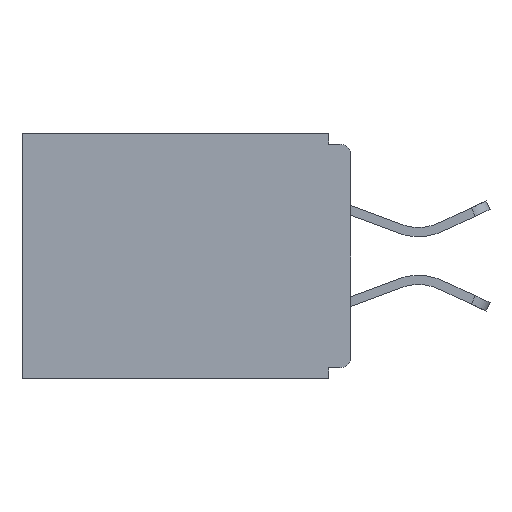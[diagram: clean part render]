
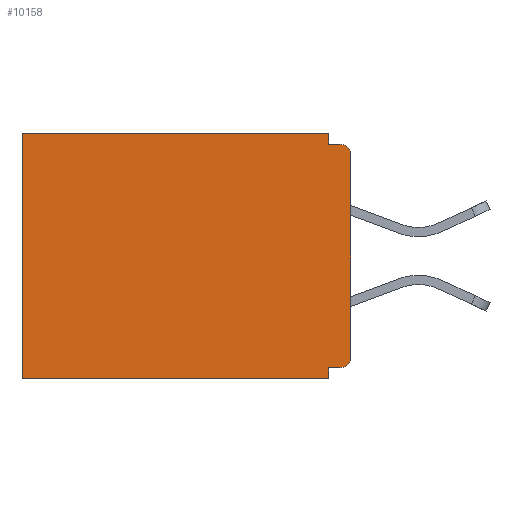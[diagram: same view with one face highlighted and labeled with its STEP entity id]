
A CAD part, left-side view. The second image highlights one B-rep face of the part: STEP entity #10158.
In plain terms, the highlighted planar face has unit normal (-1, 0, 0).
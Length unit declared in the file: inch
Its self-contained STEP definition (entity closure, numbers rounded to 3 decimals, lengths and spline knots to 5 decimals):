
#360 = CARTESIAN_POINT ( 'NONE',  ( 0.298, 0.031, -0.343 ) ) ;
#511 = VERTEX_POINT ( 'NONE', #20464 ) ;
#1311 = CARTESIAN_POINT ( 'NONE',  ( 0.298, 0., -0.328 ) ) ;
#1667 = DIRECTION ( 'NONE',  ( 1., 0., 0. ) ) ;
#1739 = CARTESIAN_POINT ( 'NONE',  ( 0.298, 0., -0.015 ) ) ;
#2010 = LINE ( 'NONE', #12875, #14584 ) ;
#2034 = VECTOR ( 'NONE', #11067, 39.37008 ) ;
#2295 = AXIS2_PLACEMENT_3D ( 'NONE', #22097, #24158, #23992 ) ;
#2498 = CARTESIAN_POINT ( 'NONE',  ( 0.298, 0.46, -0.343 ) ) ;
#2510 = FACE_OUTER_BOUND ( 'NONE', #4652, .T. ) ;
#2624 = CARTESIAN_POINT ( 'NONE',  ( 0.298, 0., -0.03 ) ) ;
#2824 = VERTEX_POINT ( 'NONE', #17046 ) ;
#2877 = LINE ( 'NONE', #1739, #2034 ) ;
#2881 = LINE ( 'NONE', #17395, #10744 ) ;
#2936 = VERTEX_POINT ( 'NONE', #21156 ) ;
#3415 = ORIENTED_EDGE ( 'NONE', *, *, #20116, .F. ) ;
#3960 = CIRCLE ( 'NONE', #19292, 0.015 ) ;
#4278 = EDGE_CURVE ( 'NONE', #511, #17230, #2881, .T. ) ;
#4652 = EDGE_LOOP ( 'NONE', ( #11288, #8865, #23082, #16800, #13172, #14732, #3415, #10312, #14212, #19176 ) ) ;
#4686 = DIRECTION ( 'NONE',  ( 0., 0., -1. ) ) ;
#5114 = VECTOR ( 'NONE', #4686, 39.37008 ) ;
#5478 = CARTESIAN_POINT ( 'NONE',  ( 0.298, 0.46, 0. ) ) ;
#5620 = VERTEX_POINT ( 'NONE', #2498 ) ;
#7881 = DIRECTION ( 'NONE',  ( 0., 0., -1. ) ) ;
#8030 = VERTEX_POINT ( 'NONE', #2624 ) ;
#8452 = CARTESIAN_POINT ( 'NONE',  ( 0.298, 0.031, -0.343 ) ) ;
#8865 = ORIENTED_EDGE ( 'NONE', *, *, #14608, .F. ) ;
#9141 = VECTOR ( 'NONE', #23404, 39.37008 ) ;
#10158 = ADVANCED_FACE ( 'NONE', ( #2510 ), #24097, .F. ) ;
#10312 = ORIENTED_EDGE ( 'NONE', *, *, #14454, .F. ) ;
#10385 = EDGE_CURVE ( 'NONE', #2936, #2824, #15359, .T. ) ;
#10394 = DIRECTION ( 'NONE',  ( 0., 1., 0. ) ) ;
#10738 = EDGE_CURVE ( 'NONE', #17230, #5620, #23297, .T. ) ;
#10744 = VECTOR ( 'NONE', #15681, 39.37008 ) ;
#11067 = DIRECTION ( 'NONE',  ( 0., -1., 0. ) ) ;
#11218 = CARTESIAN_POINT ( 'NONE',  ( 0.298, 0.031, -0.328 ) ) ;
#11288 = ORIENTED_EDGE ( 'NONE', *, *, #19928, .T. ) ;
#11345 = LINE ( 'NONE', #1311, #13118 ) ;
#11578 = DIRECTION ( 'NONE',  ( -1., 0., 0. ) ) ;
#12262 = CARTESIAN_POINT ( 'NONE',  ( 0.298, 0.46, 0. ) ) ;
#12790 = DIRECTION ( 'NONE',  ( 0., 1., 0. ) ) ;
#12806 = CARTESIAN_POINT ( 'NONE',  ( 0.298, 0., 0. ) ) ;
#12875 = CARTESIAN_POINT ( 'NONE',  ( 0.298, 0., 0. ) ) ;
#13118 = VECTOR ( 'NONE', #12790, 39.37008 ) ;
#13172 = ORIENTED_EDGE ( 'NONE', *, *, #10738, .T. ) ;
#14212 = ORIENTED_EDGE ( 'NONE', *, *, #10385, .T. ) ;
#14431 = VERTEX_POINT ( 'NONE', #23462 ) ;
#14454 = EDGE_CURVE ( 'NONE', #2936, #18669, #11345, .T. ) ;
#14584 = VECTOR ( 'NONE', #16678, 39.37008 ) ;
#14608 = EDGE_CURVE ( 'NONE', #14431, #22424, #2877, .T. ) ;
#14640 = EDGE_CURVE ( 'NONE', #8030, #2824, #2010, .T. ) ;
#14666 = CARTESIAN_POINT ( 'NONE',  ( 0.298, 0.015, -0.015 ) ) ;
#14732 = ORIENTED_EDGE ( 'NONE', *, *, #21633, .F. ) ;
#15359 = CIRCLE ( 'NONE', #2295, 0.015 ) ;
#15587 = VECTOR ( 'NONE', #10394, 39.37008 ) ;
#15681 = DIRECTION ( 'NONE',  ( 0., 1., 0. ) ) ;
#16324 = VECTOR ( 'NONE', #23312, 39.37008 ) ;
#16678 = DIRECTION ( 'NONE',  ( 0., 0., -1. ) ) ;
#16800 = ORIENTED_EDGE ( 'NONE', *, *, #4278, .T. ) ;
#17046 = CARTESIAN_POINT ( 'NONE',  ( 0.298, 0., -0.313 ) ) ;
#17230 = VERTEX_POINT ( 'NONE', #5478 ) ;
#17395 = CARTESIAN_POINT ( 'NONE',  ( 0.298, 0., 0. ) ) ;
#18319 = LINE ( 'NONE', #8452, #5114 ) ;
#18669 = VERTEX_POINT ( 'NONE', #11218 ) ;
#18917 = EDGE_CURVE ( 'NONE', #511, #14431, #21049, .T. ) ;
#19176 = ORIENTED_EDGE ( 'NONE', *, *, #14640, .F. ) ;
#19292 = AXIS2_PLACEMENT_3D ( 'NONE', #22858, #11578, #7881 ) ;
#19928 = EDGE_CURVE ( 'NONE', #8030, #22424, #3960, .T. ) ;
#20013 = LINE ( 'NONE', #21851, #15587 ) ;
#20116 = EDGE_CURVE ( 'NONE', #18669, #21412, #18319, .T. ) ;
#20464 = CARTESIAN_POINT ( 'NONE',  ( 0.298, 0.031, 0. ) ) ;
#21049 = LINE ( 'NONE', #23556, #16324 ) ;
#21156 = CARTESIAN_POINT ( 'NONE',  ( 0.298, 0.015, -0.328 ) ) ;
#21412 = VERTEX_POINT ( 'NONE', #360 ) ;
#21427 = AXIS2_PLACEMENT_3D ( 'NONE', #12806, #1667, #22289 ) ;
#21633 = EDGE_CURVE ( 'NONE', #21412, #5620, #20013, .T. ) ;
#21851 = CARTESIAN_POINT ( 'NONE',  ( 0.298, 0., -0.343 ) ) ;
#22097 = CARTESIAN_POINT ( 'NONE',  ( 0.298, 0.015, -0.313 ) ) ;
#22289 = DIRECTION ( 'NONE',  ( 0., 0., -1. ) ) ;
#22424 = VERTEX_POINT ( 'NONE', #14666 ) ;
#22858 = CARTESIAN_POINT ( 'NONE',  ( 0.298, 0.015, -0.03 ) ) ;
#23082 = ORIENTED_EDGE ( 'NONE', *, *, #18917, .F. ) ;
#23297 = LINE ( 'NONE', #12262, #9141 ) ;
#23312 = DIRECTION ( 'NONE',  ( 0., 0., -1. ) ) ;
#23404 = DIRECTION ( 'NONE',  ( 0., 0., -1. ) ) ;
#23462 = CARTESIAN_POINT ( 'NONE',  ( 0.298, 0.031, -0.015 ) ) ;
#23556 = CARTESIAN_POINT ( 'NONE',  ( 0.298, 0.031, -0.343 ) ) ;
#23992 = DIRECTION ( 'NONE',  ( 0., 0., -1. ) ) ;
#24097 = PLANE ( 'NONE',  #21427 ) ;
#24158 = DIRECTION ( 'NONE',  ( -1., 0., 0. ) ) ;
